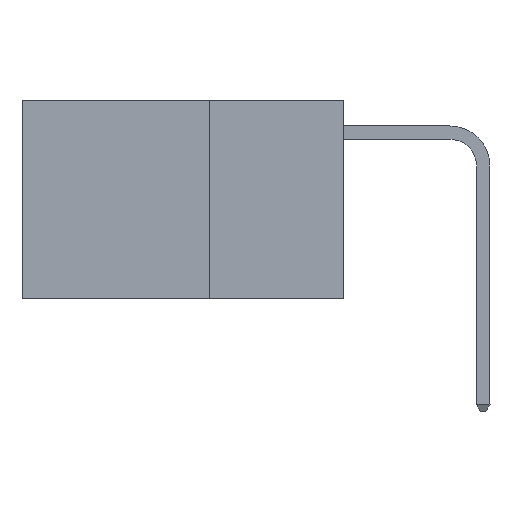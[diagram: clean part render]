
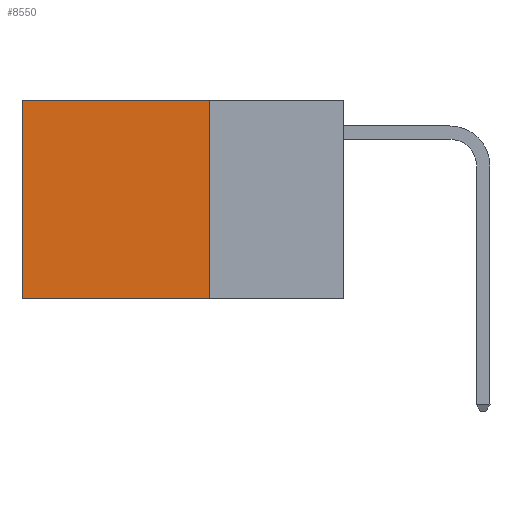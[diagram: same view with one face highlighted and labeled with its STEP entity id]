
A CAD part, left-side view. The second image highlights one B-rep face of the part: STEP entity #8550.
In plain terms, the highlighted planar face has unit normal (-1, 0, 0).
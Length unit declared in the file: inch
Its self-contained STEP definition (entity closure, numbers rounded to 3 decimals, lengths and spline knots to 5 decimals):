
#150 = EDGE_CURVE ( 'NONE', #4604, #5758, #6187, .T. ) ;
#312 = CARTESIAN_POINT ( 'NONE',  ( 0.2625, 0.6, 0. ) ) ;
#554 = VECTOR ( 'NONE', #11943, 39.37008 ) ;
#599 = LINE ( 'NONE', #11932, #554 ) ;
#758 = ORIENTED_EDGE ( 'NONE', *, *, #11066, .T. ) ;
#797 = EDGE_LOOP ( 'NONE', ( #758, #1478, #12072, #11495 ) ) ;
#1113 = DIRECTION ( 'NONE',  ( 0., 1., 0. ) ) ;
#1353 = CARTESIAN_POINT ( 'NONE',  ( 0.2625, 0.25, -0.37 ) ) ;
#1478 = ORIENTED_EDGE ( 'NONE', *, *, #9082, .F. ) ;
#1622 = VECTOR ( 'NONE', #1113, 39.37008 ) ;
#1725 = LINE ( 'NONE', #1353, #1622 ) ;
#1868 = VERTEX_POINT ( 'NONE', #2672 ) ;
#2672 = CARTESIAN_POINT ( 'NONE',  ( 0.2625, 0.6, -0.37 ) ) ;
#3727 = EDGE_CURVE ( 'NONE', #4604, #10059, #599, .T. ) ;
#3942 = VECTOR ( 'NONE', #7227, 39.37008 ) ;
#4088 = CARTESIAN_POINT ( 'NONE',  ( 0.2625, 0.6, 0. ) ) ;
#4151 = AXIS2_PLACEMENT_3D ( 'NONE', #10890, #10842, #10833 ) ;
#4604 = VERTEX_POINT ( 'NONE', #5528 ) ;
#5528 = CARTESIAN_POINT ( 'NONE',  ( 0.2625, 0.25, 0. ) ) ;
#5758 = VERTEX_POINT ( 'NONE', #4088 ) ;
#6187 = LINE ( 'NONE', #9913, #7048 ) ;
#6591 = LINE ( 'NONE', #312, #3942 ) ;
#7048 = VECTOR ( 'NONE', #9862, 39.37008 ) ;
#7227 = DIRECTION ( 'NONE',  ( 0., 0., -1. ) ) ;
#8550 = ADVANCED_FACE ( 'NONE', ( #10782 ), #10923, .F. ) ;
#9082 = EDGE_CURVE ( 'NONE', #10059, #1868, #1725, .T. ) ;
#9862 = DIRECTION ( 'NONE',  ( 0., 1., 0. ) ) ;
#9913 = CARTESIAN_POINT ( 'NONE',  ( 0.2625, 0.25, 0. ) ) ;
#10059 = VERTEX_POINT ( 'NONE', #13647 ) ;
#10782 = FACE_OUTER_BOUND ( 'NONE', #797, .T. ) ;
#10833 = DIRECTION ( 'NONE',  ( 0., 0., -1. ) ) ;
#10842 = DIRECTION ( 'NONE',  ( 1., 0., 0. ) ) ;
#10890 = CARTESIAN_POINT ( 'NONE',  ( 0.2625, 0.25, 0. ) ) ;
#10923 = PLANE ( 'NONE',  #4151 ) ;
#11066 = EDGE_CURVE ( 'NONE', #5758, #1868, #6591, .T. ) ;
#11495 = ORIENTED_EDGE ( 'NONE', *, *, #150, .T. ) ;
#11932 = CARTESIAN_POINT ( 'NONE',  ( 0.2625, 0.25, 0. ) ) ;
#11943 = DIRECTION ( 'NONE',  ( 0., 0., -1. ) ) ;
#12072 = ORIENTED_EDGE ( 'NONE', *, *, #3727, .F. ) ;
#13647 = CARTESIAN_POINT ( 'NONE',  ( 0.2625, 0.25, -0.37 ) ) ;
